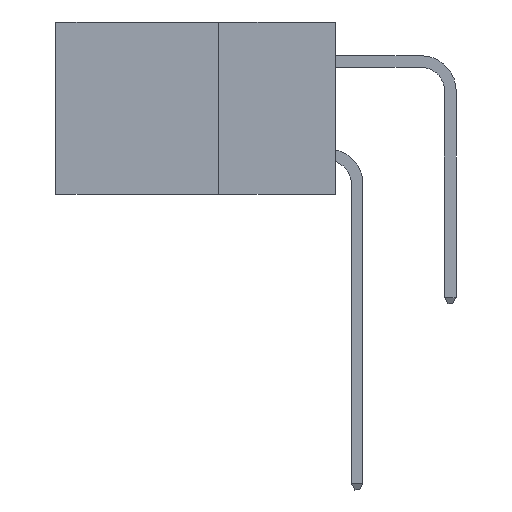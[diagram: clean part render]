
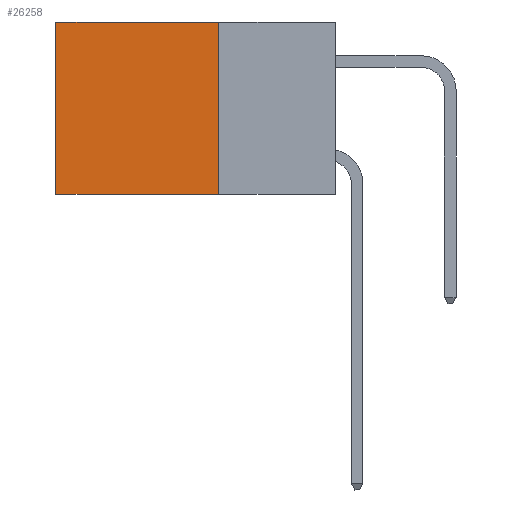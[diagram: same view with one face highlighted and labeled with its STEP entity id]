
A CAD part, left-side view. The second image highlights one B-rep face of the part: STEP entity #26258.
In plain terms, the highlighted planar face has unit normal (-1, 0, 0).
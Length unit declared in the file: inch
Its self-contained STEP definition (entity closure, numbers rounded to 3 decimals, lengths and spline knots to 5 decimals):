
#77 = FACE_OUTER_BOUND ( 'NONE', #17758, .T. ) ;
#211 = AXIS2_PLACEMENT_3D ( 'NONE', #12329, #10126, #16943 ) ;
#1093 = EDGE_CURVE ( 'NONE', #3036, #4762, #24003, .T. ) ;
#2586 = EDGE_CURVE ( 'NONE', #4762, #4090, #13413, .T. ) ;
#2978 = ORIENTED_EDGE ( 'NONE', *, *, #20465, .F. ) ;
#3036 = VERTEX_POINT ( 'NONE', #4642 ) ;
#3175 = DIRECTION ( 'NONE',  ( 0., 0., -1. ) ) ;
#3445 = CARTESIAN_POINT ( 'NONE',  ( 0.2875, 0.25, -0.37 ) ) ;
#3557 = CARTESIAN_POINT ( 'NONE',  ( 0.2875, 0.6, 0. ) ) ;
#3695 = DIRECTION ( 'NONE',  ( 0., 1., 0. ) ) ;
#3933 = ORIENTED_EDGE ( 'NONE', *, *, #1093, .T. ) ;
#4090 = VERTEX_POINT ( 'NONE', #19465 ) ;
#4642 = CARTESIAN_POINT ( 'NONE',  ( 0.2875, 0.25, 0. ) ) ;
#4751 = CARTESIAN_POINT ( 'NONE',  ( 0.2875, 0.25, 0. ) ) ;
#4762 = VERTEX_POINT ( 'NONE', #7039 ) ;
#5253 = VECTOR ( 'NONE', #3175, 39.37008 ) ;
#5411 = VERTEX_POINT ( 'NONE', #3445 ) ;
#6644 = CARTESIAN_POINT ( 'NONE',  ( 0.2875, 0.25, 0. ) ) ;
#7039 = CARTESIAN_POINT ( 'NONE',  ( 0.2875, 0.6, 0. ) ) ;
#8406 = EDGE_CURVE ( 'NONE', #5411, #4090, #9103, .T. ) ;
#9103 = LINE ( 'NONE', #16632, #25753 ) ;
#10126 = DIRECTION ( 'NONE',  ( 1., 0., 0. ) ) ;
#10429 = VECTOR ( 'NONE', #12863, 39.37008 ) ;
#12329 = CARTESIAN_POINT ( 'NONE',  ( 0.2875, 0.25, 0. ) ) ;
#12863 = DIRECTION ( 'NONE',  ( 0., 0., -1. ) ) ;
#13413 = LINE ( 'NONE', #3557, #5253 ) ;
#16187 = LINE ( 'NONE', #6644, #10429 ) ;
#16632 = CARTESIAN_POINT ( 'NONE',  ( 0.2875, 0.25, -0.37 ) ) ;
#16943 = DIRECTION ( 'NONE',  ( 0., 0., -1. ) ) ;
#17758 = EDGE_LOOP ( 'NONE', ( #23260, #23781, #2978, #3933 ) ) ;
#19054 = PLANE ( 'NONE',  #211 ) ;
#19465 = CARTESIAN_POINT ( 'NONE',  ( 0.2875, 0.6, -0.37 ) ) ;
#20465 = EDGE_CURVE ( 'NONE', #3036, #5411, #16187, .T. ) ;
#23260 = ORIENTED_EDGE ( 'NONE', *, *, #2586, .T. ) ;
#23662 = VECTOR ( 'NONE', #24461, 39.37008 ) ;
#23781 = ORIENTED_EDGE ( 'NONE', *, *, #8406, .F. ) ;
#24003 = LINE ( 'NONE', #4751, #23662 ) ;
#24461 = DIRECTION ( 'NONE',  ( 0., 1., 0. ) ) ;
#25753 = VECTOR ( 'NONE', #3695, 39.37008 ) ;
#26258 = ADVANCED_FACE ( 'NONE', ( #77 ), #19054, .F. ) ;
